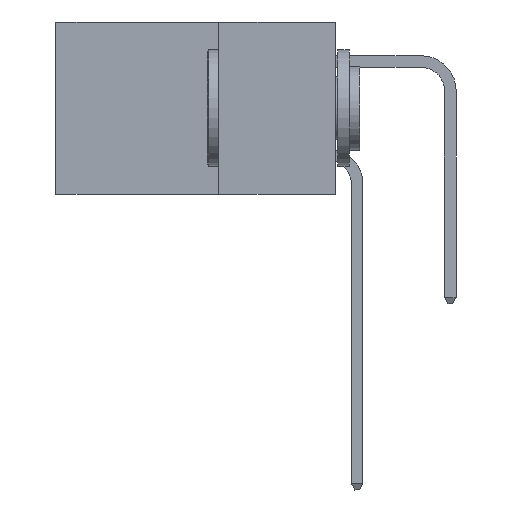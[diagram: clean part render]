
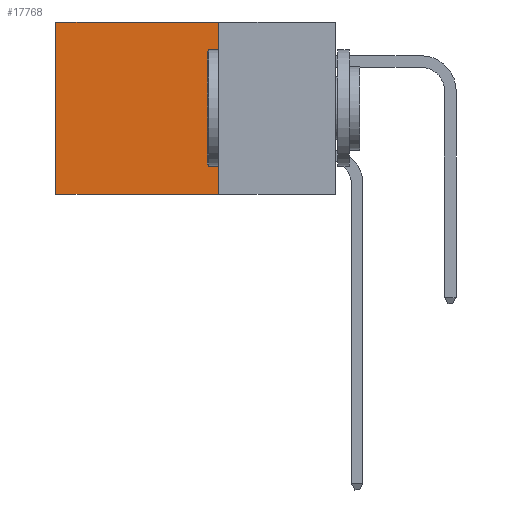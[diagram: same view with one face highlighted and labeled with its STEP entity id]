
A CAD part, left-side view. The second image highlights one B-rep face of the part: STEP entity #17768.
In plain terms, the highlighted planar face has unit normal (-1, 0, 0).
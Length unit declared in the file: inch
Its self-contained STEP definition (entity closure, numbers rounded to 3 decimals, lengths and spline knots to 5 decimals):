
#1189 = VECTOR ( 'NONE', #22030, 39.37008 ) ;
#1925 = VERTEX_POINT ( 'NONE', #12762 ) ;
#2309 = ORIENTED_EDGE ( 'NONE', *, *, #25496, .F. ) ;
#2435 = CARTESIAN_POINT ( 'NONE',  ( 0.2875, 0.25, -0.37 ) ) ;
#3150 = VECTOR ( 'NONE', #4083, 39.37008 ) ;
#4083 = DIRECTION ( 'NONE',  ( 0., 1., 0. ) ) ;
#4265 = CARTESIAN_POINT ( 'NONE',  ( 0.2875, 0.25, 0. ) ) ;
#4614 = CARTESIAN_POINT ( 'NONE',  ( 0.2875, 0.25, -0.37 ) ) ;
#5309 = EDGE_CURVE ( 'NONE', #15994, #24920, #7333, .T. ) ;
#5514 = ORIENTED_EDGE ( 'NONE', *, *, #27678, .T. ) ;
#6456 = DIRECTION ( 'NONE',  ( 0., 1., 0. ) ) ;
#7096 = LINE ( 'NONE', #4265, #1189 ) ;
#7333 = LINE ( 'NONE', #2435, #3150 ) ;
#7915 = CARTESIAN_POINT ( 'NONE',  ( 0.2875, 0.6, 0. ) ) ;
#7959 = DIRECTION ( 'NONE',  ( 0., 0., -1. ) ) ;
#9907 = CARTESIAN_POINT ( 'NONE',  ( 0.2875, 0.6, 0. ) ) ;
#10115 = CARTESIAN_POINT ( 'NONE',  ( 0.2875, 0.6, -0.37 ) ) ;
#12059 = LINE ( 'NONE', #9907, #24584 ) ;
#12762 = CARTESIAN_POINT ( 'NONE',  ( 0.2875, 0.25, 0. ) ) ;
#12840 = ORIENTED_EDGE ( 'NONE', *, *, #16864, .T. ) ;
#15994 = VERTEX_POINT ( 'NONE', #4614 ) ;
#16525 = FACE_OUTER_BOUND ( 'NONE', #24097, .T. ) ;
#16864 = EDGE_CURVE ( 'NONE', #21696, #24920, #12059, .T. ) ;
#17205 = DIRECTION ( 'NONE',  ( 0., 0., -1. ) ) ;
#17382 = CARTESIAN_POINT ( 'NONE',  ( 0.2875, 0.25, 0. ) ) ;
#17768 = ADVANCED_FACE ( 'NONE', ( #16525 ), #23857, .F. ) ;
#19677 = CARTESIAN_POINT ( 'NONE',  ( 0.2875, 0.25, 0. ) ) ;
#20541 = VECTOR ( 'NONE', #6456, 39.37008 ) ;
#21696 = VERTEX_POINT ( 'NONE', #7915 ) ;
#22030 = DIRECTION ( 'NONE',  ( 0., 0., -1. ) ) ;
#23422 = ORIENTED_EDGE ( 'NONE', *, *, #5309, .F. ) ;
#23857 = PLANE ( 'NONE',  #26399 ) ;
#24038 = DIRECTION ( 'NONE',  ( 1., 0., 0. ) ) ;
#24097 = EDGE_LOOP ( 'NONE', ( #12840, #23422, #2309, #5514 ) ) ;
#24584 = VECTOR ( 'NONE', #7959, 39.37008 ) ;
#24920 = VERTEX_POINT ( 'NONE', #10115 ) ;
#25496 = EDGE_CURVE ( 'NONE', #1925, #15994, #7096, .T. ) ;
#26399 = AXIS2_PLACEMENT_3D ( 'NONE', #19677, #24038, #17205 ) ;
#27163 = LINE ( 'NONE', #17382, #20541 ) ;
#27678 = EDGE_CURVE ( 'NONE', #1925, #21696, #27163, .T. ) ;
